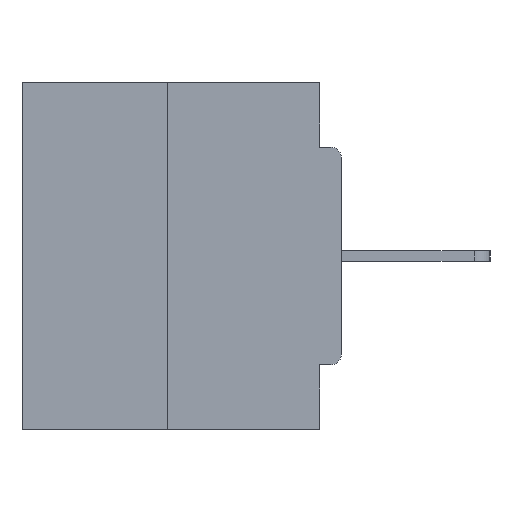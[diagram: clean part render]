
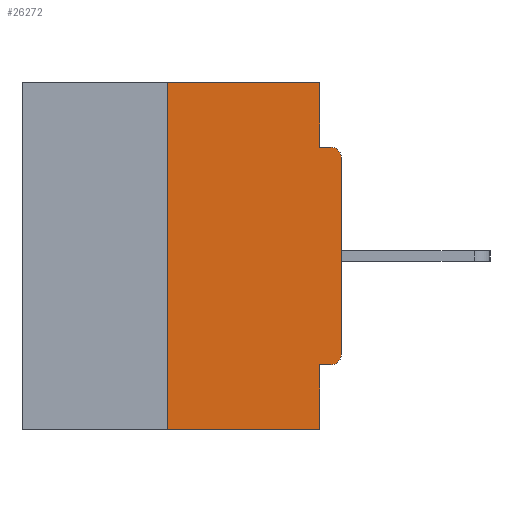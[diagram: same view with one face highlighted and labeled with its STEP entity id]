
A CAD part, left-side view. The second image highlights one B-rep face of the part: STEP entity #26272.
In plain terms, the highlighted planar face has unit normal (-1, 0, 0).
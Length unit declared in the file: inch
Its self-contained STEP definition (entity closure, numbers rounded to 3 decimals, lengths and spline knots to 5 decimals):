
#185 = DIRECTION ( 'NONE',  ( -1., 0., 0. ) ) ;
#236 = VECTOR ( 'NONE', #26827, 39.37008 ) ;
#410 = CARTESIAN_POINT ( 'NONE',  ( 0., 0.031, -0.5 ) ) ;
#669 = ORIENTED_EDGE ( 'NONE', *, *, #18737, .F. ) ;
#731 = VERTEX_POINT ( 'NONE', #3040 ) ;
#753 = CARTESIAN_POINT ( 'NONE',  ( 0., 0., -0.3915 ) ) ;
#1016 = CARTESIAN_POINT ( 'NONE',  ( 0., 0.031, 0. ) ) ;
#1303 = AXIS2_PLACEMENT_3D ( 'NONE', #19922, #185, #8788 ) ;
#1910 = CARTESIAN_POINT ( 'NONE',  ( 0., 0.031, -0.4065 ) ) ;
#2001 = ORIENTED_EDGE ( 'NONE', *, *, #17929, .T. ) ;
#2167 = VECTOR ( 'NONE', #9567, 39.37008 ) ;
#2316 = VERTEX_POINT ( 'NONE', #13747 ) ;
#2694 = FACE_OUTER_BOUND ( 'NONE', #26233, .T. ) ;
#2781 = CARTESIAN_POINT ( 'NONE',  ( 0., 0.015, -0.1085 ) ) ;
#3016 = CARTESIAN_POINT ( 'NONE',  ( 0., 0., -0.0935 ) ) ;
#3040 = CARTESIAN_POINT ( 'NONE',  ( 0., 0.031, -0.5 ) ) ;
#3509 = DIRECTION ( 'NONE',  ( 0., -1., 0. ) ) ;
#3598 = CARTESIAN_POINT ( 'NONE',  ( 0., 0., -0.1085 ) ) ;
#3632 = VECTOR ( 'NONE', #9307, 39.37008 ) ;
#4007 = VERTEX_POINT ( 'NONE', #25241 ) ;
#4884 = CARTESIAN_POINT ( 'NONE',  ( 0., 0., -0.4065 ) ) ;
#5068 = AXIS2_PLACEMENT_3D ( 'NONE', #2781, #20646, #7612 ) ;
#5134 = PLANE ( 'NONE',  #21008 ) ;
#5655 = LINE ( 'NONE', #11671, #236 ) ;
#5683 = DIRECTION ( 'NONE',  ( 0., -1., 0. ) ) ;
#5792 = CARTESIAN_POINT ( 'NONE',  ( 0., 0.015, -0.0935 ) ) ;
#5911 = EDGE_CURVE ( 'NONE', #18502, #731, #22730, .T. ) ;
#6217 = CARTESIAN_POINT ( 'NONE',  ( 0., 0.031, -0.0935 ) ) ;
#7612 = DIRECTION ( 'NONE',  ( 0., 0., -1. ) ) ;
#8788 = DIRECTION ( 'NONE',  ( 0., 0., -1. ) ) ;
#9291 = DIRECTION ( 'NONE',  ( 0., 0., 1. ) ) ;
#9307 = DIRECTION ( 'NONE',  ( 0., 1., 0. ) ) ;
#9391 = VERTEX_POINT ( 'NONE', #11704 ) ;
#9567 = DIRECTION ( 'NONE',  ( 0., 0., -1. ) ) ;
#9947 = ORIENTED_EDGE ( 'NONE', *, *, #22534, .F. ) ;
#10156 = VECTOR ( 'NONE', #27207, 39.37008 ) ;
#10906 = ORIENTED_EDGE ( 'NONE', *, *, #5911, .F. ) ;
#11432 = LINE ( 'NONE', #20148, #16961 ) ;
#11650 = VERTEX_POINT ( 'NONE', #5792 ) ;
#11671 = CARTESIAN_POINT ( 'NONE',  ( 0., 0.25, 0. ) ) ;
#11704 = CARTESIAN_POINT ( 'NONE',  ( 0., 0.015, -0.4065 ) ) ;
#11744 = DIRECTION ( 'NONE',  ( 0., -1., 0. ) ) ;
#13275 = DIRECTION ( 'NONE',  ( 1., 0., 0. ) ) ;
#13747 = CARTESIAN_POINT ( 'NONE',  ( 0., 0.031, 0. ) ) ;
#13892 = LINE ( 'NONE', #3016, #16463 ) ;
#13988 = CARTESIAN_POINT ( 'NONE',  ( 0., 0.46, -0.5 ) ) ;
#14545 = CARTESIAN_POINT ( 'NONE',  ( 0., 0.25, 0. ) ) ;
#15736 = VECTOR ( 'NONE', #3509, 39.37008 ) ;
#16463 = VECTOR ( 'NONE', #11744, 39.37008 ) ;
#16784 = VERTEX_POINT ( 'NONE', #6217 ) ;
#16961 = VECTOR ( 'NONE', #9291, 39.37008 ) ;
#17086 = EDGE_CURVE ( 'NONE', #18836, #11650, #23789, .T. ) ;
#17695 = CARTESIAN_POINT ( 'NONE',  ( 0., 0.46, 0. ) ) ;
#17929 = EDGE_CURVE ( 'NONE', #26684, #18836, #11432, .T. ) ;
#18413 = LINE ( 'NONE', #13988, #27413 ) ;
#18502 = VERTEX_POINT ( 'NONE', #1910 ) ;
#18659 = CIRCLE ( 'NONE', #1303, 0.015 ) ;
#18730 = ORIENTED_EDGE ( 'NONE', *, *, #25748, .F. ) ;
#18737 = EDGE_CURVE ( 'NONE', #2316, #16784, #20609, .T. ) ;
#18836 = VERTEX_POINT ( 'NONE', #3598 ) ;
#19843 = ORIENTED_EDGE ( 'NONE', *, *, #17086, .T. ) ;
#19922 = CARTESIAN_POINT ( 'NONE',  ( 0., 0.015, -0.3915 ) ) ;
#20148 = CARTESIAN_POINT ( 'NONE',  ( 0., 0., 0. ) ) ;
#20609 = LINE ( 'NONE', #1016, #10156 ) ;
#20646 = DIRECTION ( 'NONE',  ( -1., 0., 0. ) ) ;
#20887 = VERTEX_POINT ( 'NONE', #14545 ) ;
#21008 = AXIS2_PLACEMENT_3D ( 'NONE', #17695, #13275, #24570 ) ;
#21274 = EDGE_CURVE ( 'NONE', #20887, #2316, #25824, .T. ) ;
#22178 = LINE ( 'NONE', #4884, #3632 ) ;
#22534 = EDGE_CURVE ( 'NONE', #4007, #20887, #5655, .T. ) ;
#22730 = LINE ( 'NONE', #410, #2167 ) ;
#23098 = CARTESIAN_POINT ( 'NONE',  ( 0., 0.46, 0. ) ) ;
#23789 = CIRCLE ( 'NONE', #5068, 0.015 ) ;
#24570 = DIRECTION ( 'NONE',  ( 0., 0., -1. ) ) ;
#25170 = EDGE_CURVE ( 'NONE', #9391, #26684, #18659, .T. ) ;
#25241 = CARTESIAN_POINT ( 'NONE',  ( 0., 0.25, -0.5 ) ) ;
#25748 = EDGE_CURVE ( 'NONE', #9391, #18502, #22178, .T. ) ;
#25824 = LINE ( 'NONE', #23098, #15736 ) ;
#26083 = ORIENTED_EDGE ( 'NONE', *, *, #25170, .T. ) ;
#26233 = EDGE_LOOP ( 'NONE', ( #27869, #9947, #26642, #10906, #18730, #26083, #2001, #19843, #28240, #669 ) ) ;
#26272 = ADVANCED_FACE ( 'NONE', ( #2694 ), #5134, .F. ) ;
#26326 = EDGE_CURVE ( 'NONE', #4007, #731, #18413, .T. ) ;
#26642 = ORIENTED_EDGE ( 'NONE', *, *, #26326, .T. ) ;
#26684 = VERTEX_POINT ( 'NONE', #753 ) ;
#26827 = DIRECTION ( 'NONE',  ( 0., 0., 1. ) ) ;
#27124 = EDGE_CURVE ( 'NONE', #16784, #11650, #13892, .T. ) ;
#27207 = DIRECTION ( 'NONE',  ( 0., 0., -1. ) ) ;
#27413 = VECTOR ( 'NONE', #5683, 39.37008 ) ;
#27869 = ORIENTED_EDGE ( 'NONE', *, *, #21274, .F. ) ;
#28240 = ORIENTED_EDGE ( 'NONE', *, *, #27124, .F. ) ;
